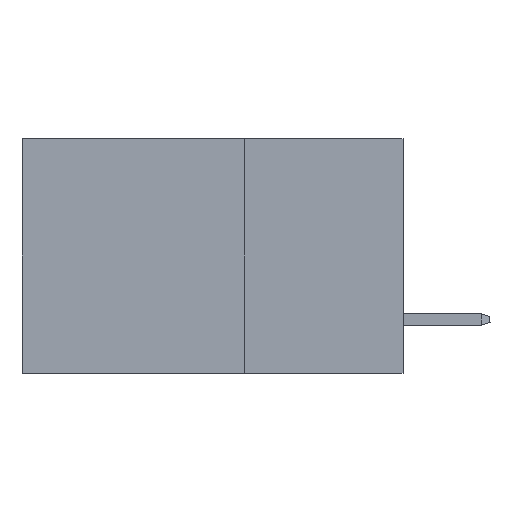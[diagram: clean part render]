
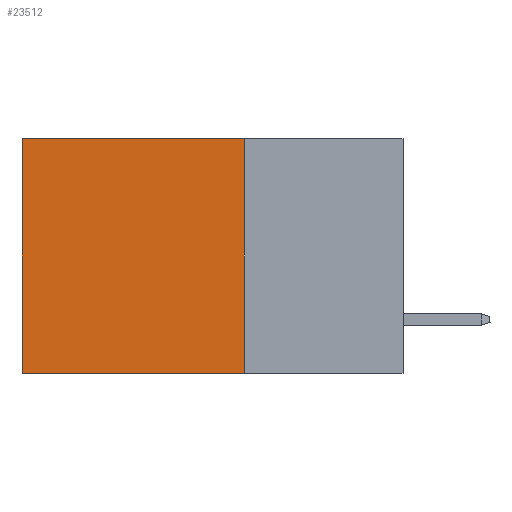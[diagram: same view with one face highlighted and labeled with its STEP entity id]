
A CAD part, left-side view. The second image highlights one B-rep face of the part: STEP entity #23512.
In plain terms, the highlighted planar face has unit normal (-1, 0, 0).
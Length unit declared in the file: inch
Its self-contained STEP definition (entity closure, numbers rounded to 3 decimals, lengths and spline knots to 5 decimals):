
#99 = FACE_OUTER_BOUND ( 'NONE', #9116, .T. ) ;
#2393 = CARTESIAN_POINT ( 'NONE',  ( 0.2875, 0.6, 0. ) ) ;
#2645 = EDGE_CURVE ( 'NONE', #9924, #28476, #15998, .T. ) ;
#3880 = CARTESIAN_POINT ( 'NONE',  ( 0.2875, 0.6, 0. ) ) ;
#4337 = DIRECTION ( 'NONE',  ( 0., 0., -1. ) ) ;
#4710 = LINE ( 'NONE', #23716, #6147 ) ;
#4945 = CARTESIAN_POINT ( 'NONE',  ( 0.2875, 0.25, 0. ) ) ;
#5295 = ORIENTED_EDGE ( 'NONE', *, *, #28758, .F. ) ;
#6147 = VECTOR ( 'NONE', #14511, 39.37008 ) ;
#6174 = VERTEX_POINT ( 'NONE', #27260 ) ;
#6701 = DIRECTION ( 'NONE',  ( 1., 0., 0. ) ) ;
#9091 = VECTOR ( 'NONE', #4337, 39.37008 ) ;
#9116 = EDGE_LOOP ( 'NONE', ( #12711, #5295, #23284, #20166 ) ) ;
#9254 = DIRECTION ( 'NONE',  ( 0., 0., -1. ) ) ;
#9684 = VECTOR ( 'NONE', #10978, 39.37008 ) ;
#9924 = VERTEX_POINT ( 'NONE', #4945 ) ;
#10885 = LINE ( 'NONE', #13168, #12231 ) ;
#10978 = DIRECTION ( 'NONE',  ( 0., 1., 0. ) ) ;
#11530 = EDGE_CURVE ( 'NONE', #28476, #6174, #29500, .T. ) ;
#12231 = VECTOR ( 'NONE', #22402, 39.37008 ) ;
#12711 = ORIENTED_EDGE ( 'NONE', *, *, #11530, .T. ) ;
#13168 = CARTESIAN_POINT ( 'NONE',  ( 0.2875, 0.25, -0.37 ) ) ;
#14492 = AXIS2_PLACEMENT_3D ( 'NONE', #27380, #6701, #9254 ) ;
#14511 = DIRECTION ( 'NONE',  ( 0., 0., -1. ) ) ;
#15998 = LINE ( 'NONE', #20666, #9684 ) ;
#20166 = ORIENTED_EDGE ( 'NONE', *, *, #2645, .T. ) ;
#20666 = CARTESIAN_POINT ( 'NONE',  ( 0.2875, 0.25, 0. ) ) ;
#22104 = EDGE_CURVE ( 'NONE', #9924, #25938, #4710, .T. ) ;
#22402 = DIRECTION ( 'NONE',  ( 0., 1., 0. ) ) ;
#23284 = ORIENTED_EDGE ( 'NONE', *, *, #22104, .F. ) ;
#23512 = ADVANCED_FACE ( 'NONE', ( #99 ), #27693, .F. ) ;
#23716 = CARTESIAN_POINT ( 'NONE',  ( 0.2875, 0.25, 0. ) ) ;
#25938 = VERTEX_POINT ( 'NONE', #27687 ) ;
#27260 = CARTESIAN_POINT ( 'NONE',  ( 0.2875, 0.6, -0.37 ) ) ;
#27380 = CARTESIAN_POINT ( 'NONE',  ( 0.2875, 0.25, 0. ) ) ;
#27687 = CARTESIAN_POINT ( 'NONE',  ( 0.2875, 0.25, -0.37 ) ) ;
#27693 = PLANE ( 'NONE',  #14492 ) ;
#28476 = VERTEX_POINT ( 'NONE', #2393 ) ;
#28758 = EDGE_CURVE ( 'NONE', #25938, #6174, #10885, .T. ) ;
#29500 = LINE ( 'NONE', #3880, #9091 ) ;
